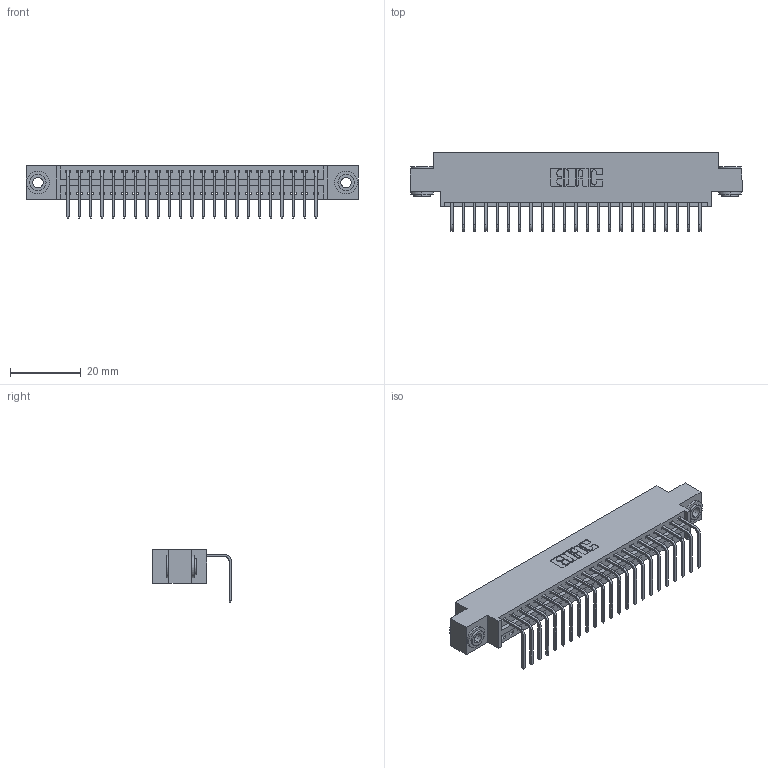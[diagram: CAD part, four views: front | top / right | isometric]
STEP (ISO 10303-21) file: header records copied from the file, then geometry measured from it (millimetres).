
FILE_DESCRIPTION (( 'STEP AP203' ), '1' );
FILE_NAME ('346-023-558-603.STEP', '2022-05-05T21:48:37', ( '' ), ( '' ), 'SwSTEP 2.0', 'SolidWorks 2020', '' );
FILE_SCHEMA (( 'CONFIG_CONTROL_DESIGN' ));
Length unit declared in the file: inch
Products named in the file (4): 346-023-558-603; 346 Part_0.170 Offset - 0.156 Dia-TH; 345-250-002_345-250-002-102; 345-292-001_558 Tail - 2
Assembly tree (26 placements, depth 2):
  346-023-558-603
    346 Part_0.170 Offset - 0.156 Dia-TH
    345-292-001_558 Tail - 2  x23
    345-250-002_345-250-002-102  x2
Bounding box: 93.6 x 22.16 x 14.73 mm (x, y, z)
Volume: 8751.9 mm3; surface area: 11602.7 mm2
Topology: 26 solids, 26 shells, 1558 faces, 4639 edges, 3058 vertices
Faces by surface type: plane 1070, cylinder 480, cone 8
Entity records: 18114 total; most frequent: CARTESIAN_POINT 3094, ORIENTED_EDGE 3042, DIRECTION 2781, EDGE_CURVE 1521, LINE 1273, VECTOR 1273, VERTEX_POINT 1010, AXIS2_PLACEMENT_3D 754
